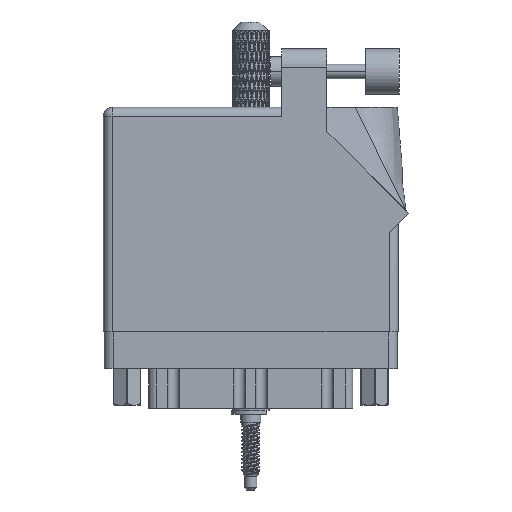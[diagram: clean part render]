
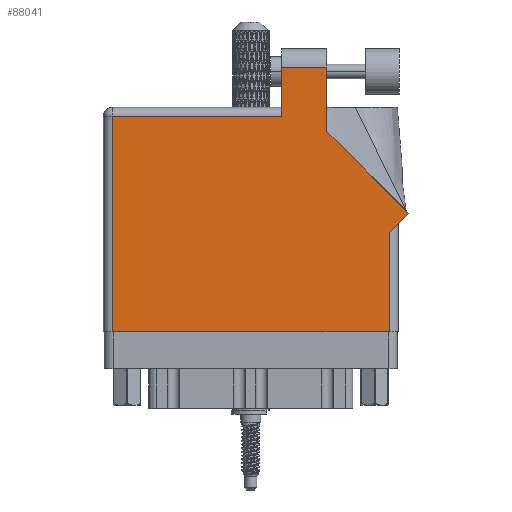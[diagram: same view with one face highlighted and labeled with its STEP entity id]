
A CAD part, front view. The second image highlights one B-rep face of the part: STEP entity #88041.
In plain terms, the highlighted face is planar.
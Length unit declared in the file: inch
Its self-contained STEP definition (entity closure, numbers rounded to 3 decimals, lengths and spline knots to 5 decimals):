
#4228 = DIRECTION ( 'NONE',  ( 0., 1., 0. ) ) ;
#6221 = VERTEX_POINT ( 'NONE', #97949 ) ;
#6644 = DIRECTION ( 'NONE',  ( 0.707, 0.707, 0. ) ) ;
#9338 = ORIENTED_EDGE ( 'NONE', *, *, #92239, .T. ) ;
#11172 = EDGE_CURVE ( 'NONE', #43082, #63267, #66057, .T. ) ;
#12857 = CARTESIAN_POINT ( 'NONE',  ( 0., 0., 0. ) ) ;
#17339 = VECTOR ( 'NONE', #4228, 39.37008 ) ;
#20442 = CARTESIAN_POINT ( 'NONE',  ( 1.948, 0., 0. ) ) ;
#21622 = EDGE_CURVE ( 'NONE', #63267, #92926, #51781, .T. ) ;
#24500 = EDGE_CURVE ( 'NONE', #33793, #6221, #39901, .T. ) ;
#24567 = CARTESIAN_POINT ( 'NONE',  ( 1.217, 1.53, 0. ) ) ;
#24590 = VERTEX_POINT ( 'NONE', #105616 ) ;
#27215 = VECTOR ( 'NONE', #43517, 39.37008 ) ;
#27545 = VECTOR ( 'NONE', #103213, 39.37008 ) ;
#31744 = DIRECTION ( 'NONE',  ( 0., -1., 0. ) ) ;
#33649 = ORIENTED_EDGE ( 'NONE', *, *, #109277, .T. ) ;
#33773 = DIRECTION ( 'NONE',  ( -1., 0., 0. ) ) ;
#33793 = VERTEX_POINT ( 'NONE', #93472 ) ;
#35377 = EDGE_CURVE ( 'NONE', #87494, #33793, #40429, .T. ) ;
#36305 = CARTESIAN_POINT ( 'NONE',  ( 1.217, 1.805, 0. ) ) ;
#39584 = AXIS2_PLACEMENT_3D ( 'NONE', #42099, #60297, #33773 ) ;
#39901 = LINE ( 'NONE', #83031, #41490 ) ;
#40429 = LINE ( 'NONE', #89121, #92945 ) ;
#41008 = DIRECTION ( 'NONE',  ( -0.707, 0.707, 0. ) ) ;
#41490 = VECTOR ( 'NONE', #41008, 39.37008 ) ;
#42099 = CARTESIAN_POINT ( 'NONE',  ( 0., 1.53, 0. ) ) ;
#42628 = FACE_OUTER_BOUND ( 'NONE', #48326, .T. ) ;
#43082 = VERTEX_POINT ( 'NONE', #56549 ) ;
#43517 = DIRECTION ( 'NONE',  ( -1., 0., 0. ) ) ;
#43708 = PLANE ( 'NONE',  #39584 ) ;
#45549 = LINE ( 'NONE', #12857, #85005 ) ;
#47908 = ORIENTED_EDGE ( 'NONE', *, *, #56659, .T. ) ;
#48027 = EDGE_CURVE ( 'NONE', #56631, #87494, #63449, .T. ) ;
#48326 = EDGE_LOOP ( 'NONE', ( #9338, #33649, #49320, #89126, #47908, #96004, #85770, #59972, #48763 ) ) ;
#48763 = ORIENTED_EDGE ( 'NONE', *, *, #24500, .T. ) ;
#49320 = ORIENTED_EDGE ( 'NONE', *, *, #11172, .T. ) ;
#51781 = LINE ( 'NONE', #78319, #27545 ) ;
#55314 = DIRECTION ( 'NONE',  ( 0., -1., 0. ) ) ;
#56229 = VECTOR ( 'NONE', #55314, 39.37008 ) ;
#56433 = VERTEX_POINT ( 'NONE', #89705 ) ;
#56549 = CARTESIAN_POINT ( 'NONE',  ( 1.217, 1.805, 0. ) ) ;
#56631 = VERTEX_POINT ( 'NONE', #20442 ) ;
#56659 = EDGE_CURVE ( 'NONE', #92926, #56433, #98411, .T. ) ;
#57557 = CARTESIAN_POINT ( 'NONE',  ( 1.524, 1.36442, 0. ) ) ;
#59972 = ORIENTED_EDGE ( 'NONE', *, *, #35377, .T. ) ;
#60297 = DIRECTION ( 'NONE',  ( 0., 0., -1. ) ) ;
#63267 = VERTEX_POINT ( 'NONE', #104401 ) ;
#63449 = LINE ( 'NONE', #87791, #17339 ) ;
#66057 = LINE ( 'NONE', #24567, #82433 ) ;
#68848 = CARTESIAN_POINT ( 'NONE',  ( 1.948, 0.675, 0. ) ) ;
#76640 = EDGE_CURVE ( 'NONE', #56433, #56631, #45549, .T. ) ;
#78319 = CARTESIAN_POINT ( 'NONE',  ( 0., 1.468, 0. ) ) ;
#80371 = DIRECTION ( 'NONE',  ( 1., 0., 0. ) ) ;
#82433 = VECTOR ( 'NONE', #31744, 39.37008 ) ;
#83031 = CARTESIAN_POINT ( 'NONE',  ( 2.08071, 0.80771, 0. ) ) ;
#85005 = VECTOR ( 'NONE', #80371, 39.37008 ) ;
#85770 = ORIENTED_EDGE ( 'NONE', *, *, #48027, .T. ) ;
#86630 = LINE ( 'NONE', #36305, #27215 ) ;
#87494 = VERTEX_POINT ( 'NONE', #68848 ) ;
#87791 = CARTESIAN_POINT ( 'NONE',  ( 1.948, 0.737, 0. ) ) ;
#88041 = ADVANCED_FACE ( 'NONE', ( #42628 ), #43708, .F. ) ;
#89121 = CARTESIAN_POINT ( 'NONE',  ( 2.01, 0.737, 0. ) ) ;
#89126 = ORIENTED_EDGE ( 'NONE', *, *, #21622, .T. ) ;
#89705 = CARTESIAN_POINT ( 'NONE',  ( 0.062, 0., 0. ) ) ;
#92183 = CARTESIAN_POINT ( 'NONE',  ( 0.062, 1.468, 0. ) ) ;
#92239 = EDGE_CURVE ( 'NONE', #6221, #24590, #92377, .T. ) ;
#92377 = LINE ( 'NONE', #57557, #107074 ) ;
#92926 = VERTEX_POINT ( 'NONE', #92183 ) ;
#92945 = VECTOR ( 'NONE', #6644, 39.37008 ) ;
#93472 = CARTESIAN_POINT ( 'NONE',  ( 2.08071, 0.80771, 0. ) ) ;
#96004 = ORIENTED_EDGE ( 'NONE', *, *, #76640, .T. ) ;
#97949 = CARTESIAN_POINT ( 'NONE',  ( 1.524, 1.36442, 0. ) ) ;
#98411 = LINE ( 'NONE', #107262, #56229 ) ;
#103213 = DIRECTION ( 'NONE',  ( -1., 0., 0. ) ) ;
#104401 = CARTESIAN_POINT ( 'NONE',  ( 1.217, 1.468, 0. ) ) ;
#105616 = CARTESIAN_POINT ( 'NONE',  ( 1.524, 1.805, 0. ) ) ;
#107074 = VECTOR ( 'NONE', #108979, 39.37008 ) ;
#107262 = CARTESIAN_POINT ( 'NONE',  ( 0.062, 0., 0. ) ) ;
#108979 = DIRECTION ( 'NONE',  ( 0., 1., 0. ) ) ;
#109277 = EDGE_CURVE ( 'NONE', #24590, #43082, #86630, .T. ) ;
